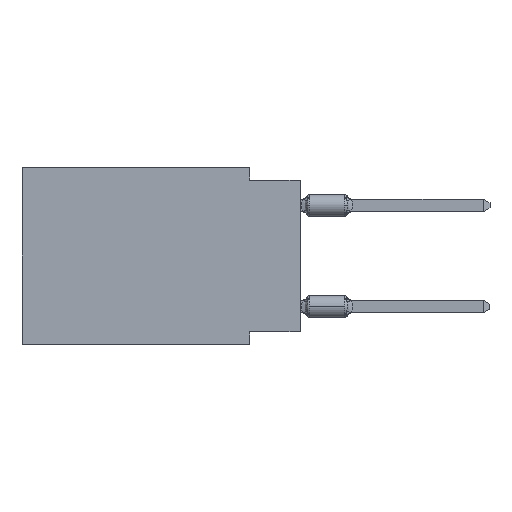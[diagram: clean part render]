
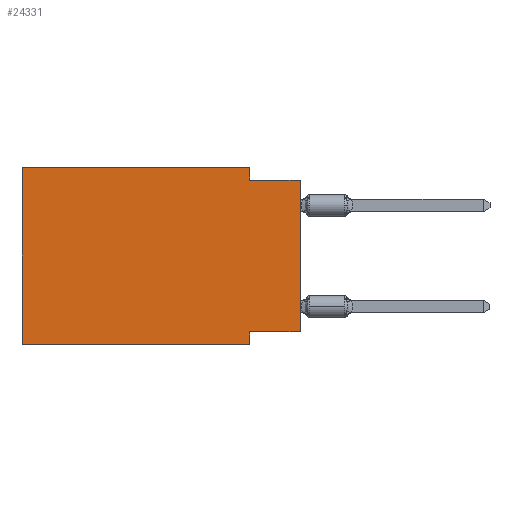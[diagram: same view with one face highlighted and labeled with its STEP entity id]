
A CAD part, left-side view. The second image highlights one B-rep face of the part: STEP entity #24331.
In plain terms, the highlighted planar face has unit normal (-1, 0, 0).
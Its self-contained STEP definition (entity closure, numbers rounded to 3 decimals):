
#382 = ORIENTED_EDGE ( 'NONE', *, *, #6302, .F. ) ;
#748 = ORIENTED_EDGE ( 'NONE', *, *, #24906, .T. ) ;
#888 = LINE ( 'NONE', #21910, #22568 ) ;
#1237 = ORIENTED_EDGE ( 'NONE', *, *, #13168, .F. ) ;
#1615 = EDGE_CURVE ( 'NONE', #13514, #8977, #14320, .T. ) ;
#1970 = ORIENTED_EDGE ( 'NONE', *, *, #20774, .F. ) ;
#3203 = CARTESIAN_POINT ( 'NONE',  ( 0., 13.97, -8.89 ) ) ;
#4067 = CARTESIAN_POINT ( 'NONE',  ( 0., 13.97, 0. ) ) ;
#4726 = ORIENTED_EDGE ( 'NONE', *, *, #1615, .F. ) ;
#5021 = CARTESIAN_POINT ( 'NONE',  ( 0., 2.54, -0.635 ) ) ;
#5173 = LINE ( 'NONE', #18449, #16795 ) ;
#6119 = VERTEX_POINT ( 'NONE', #25668 ) ;
#6302 = EDGE_CURVE ( 'NONE', #15271, #21823, #5173, .T. ) ;
#6667 = CARTESIAN_POINT ( 'NONE',  ( 0., 13.97, 0. ) ) ;
#6730 = CARTESIAN_POINT ( 'NONE',  ( 0., 13.97, -8.89 ) ) ;
#7265 = CARTESIAN_POINT ( 'NONE',  ( 0., 0., -8.255 ) ) ;
#7345 = CARTESIAN_POINT ( 'NONE',  ( 0., 2.54, 0. ) ) ;
#7660 = DIRECTION ( 'NONE',  ( 0., 0., 1. ) ) ;
#7903 = EDGE_CURVE ( 'NONE', #6119, #8271, #888, .T. ) ;
#8271 = VERTEX_POINT ( 'NONE', #8486 ) ;
#8374 = CARTESIAN_POINT ( 'NONE',  ( 0., 0., -0.635 ) ) ;
#8486 = CARTESIAN_POINT ( 'NONE',  ( 0., 2.54, -8.89 ) ) ;
#8736 = DIRECTION ( 'NONE',  ( 0., -1., 0. ) ) ;
#8977 = VERTEX_POINT ( 'NONE', #15154 ) ;
#9577 = VECTOR ( 'NONE', #11739, 1000. ) ;
#9919 = VECTOR ( 'NONE', #24692, 1000. ) ;
#10059 = VECTOR ( 'NONE', #11778, 1000. ) ;
#11593 = VERTEX_POINT ( 'NONE', #24165 ) ;
#11739 = DIRECTION ( 'NONE',  ( 0., 0., -1. ) ) ;
#11778 = DIRECTION ( 'NONE',  ( 0., -1., 0. ) ) ;
#11932 = DIRECTION ( 'NONE',  ( 1., 0., 0. ) ) ;
#12461 = ORIENTED_EDGE ( 'NONE', *, *, #7903, .F. ) ;
#13168 = EDGE_CURVE ( 'NONE', #11593, #6119, #13764, .T. ) ;
#13514 = VERTEX_POINT ( 'NONE', #5021 ) ;
#13522 = LINE ( 'NONE', #15063, #22722 ) ;
#13575 = LINE ( 'NONE', #3203, #10059 ) ;
#13725 = ORIENTED_EDGE ( 'NONE', *, *, #13980, .F. ) ;
#13764 = LINE ( 'NONE', #7265, #9919 ) ;
#13980 = EDGE_CURVE ( 'NONE', #21823, #17506, #17451, .T. ) ;
#13997 = DIRECTION ( 'NONE',  ( 0., 0., -1. ) ) ;
#14320 = LINE ( 'NONE', #8374, #18421 ) ;
#15063 = CARTESIAN_POINT ( 'NONE',  ( 0., 0., 0. ) ) ;
#15154 = CARTESIAN_POINT ( 'NONE',  ( 0., 0., -0.635 ) ) ;
#15271 = VERTEX_POINT ( 'NONE', #6730 ) ;
#15435 = DIRECTION ( 'NONE',  ( 0., 0., -1. ) ) ;
#16087 = FACE_OUTER_BOUND ( 'NONE', #20436, .T. ) ;
#16598 = VECTOR ( 'NONE', #8736, 1000. ) ;
#16795 = VECTOR ( 'NONE', #7660, 1000. ) ;
#17451 = LINE ( 'NONE', #6667, #16598 ) ;
#17506 = VERTEX_POINT ( 'NONE', #7345 ) ;
#18086 = ORIENTED_EDGE ( 'NONE', *, *, #22092, .T. ) ;
#18421 = VECTOR ( 'NONE', #22763, 1000. ) ;
#18449 = CARTESIAN_POINT ( 'NONE',  ( 0., 13.97, 0. ) ) ;
#19485 = DIRECTION ( 'NONE',  ( 0., 0., 1. ) ) ;
#20436 = EDGE_LOOP ( 'NONE', ( #748, #4726, #1970, #13725, #382, #18086, #12461, #1237 ) ) ;
#20506 = CARTESIAN_POINT ( 'NONE',  ( 0., 13.97, 0. ) ) ;
#20774 = EDGE_CURVE ( 'NONE', #17506, #13514, #27089, .T. ) ;
#21823 = VERTEX_POINT ( 'NONE', #4067 ) ;
#21910 = CARTESIAN_POINT ( 'NONE',  ( 0., 2.54, -8.89 ) ) ;
#22092 = EDGE_CURVE ( 'NONE', #15271, #8271, #13575, .T. ) ;
#22568 = VECTOR ( 'NONE', #15435, 1000. ) ;
#22722 = VECTOR ( 'NONE', #19485, 1000. ) ;
#22763 = DIRECTION ( 'NONE',  ( 0., -1., 0. ) ) ;
#24165 = CARTESIAN_POINT ( 'NONE',  ( 0., 0., -8.255 ) ) ;
#24331 = ADVANCED_FACE ( 'NONE', ( #16087 ), #26458, .F. ) ;
#24692 = DIRECTION ( 'NONE',  ( 0., 1., 0. ) ) ;
#24906 = EDGE_CURVE ( 'NONE', #11593, #8977, #13522, .T. ) ;
#25668 = CARTESIAN_POINT ( 'NONE',  ( 0., 2.54, -8.255 ) ) ;
#26293 = AXIS2_PLACEMENT_3D ( 'NONE', #20506, #11932, #13997 ) ;
#26458 = PLANE ( 'NONE',  #26293 ) ;
#26542 = CARTESIAN_POINT ( 'NONE',  ( 0., 2.54, 0. ) ) ;
#27089 = LINE ( 'NONE', #26542, #9577 ) ;
